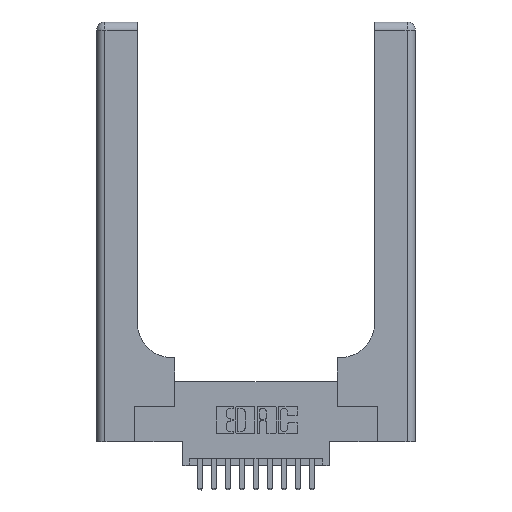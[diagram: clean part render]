
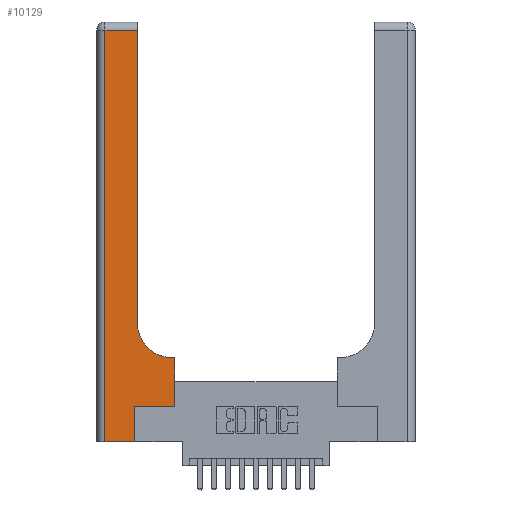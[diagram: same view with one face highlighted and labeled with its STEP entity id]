
A CAD part, top view. The second image highlights one B-rep face of the part: STEP entity #10129.
In plain terms, the highlighted planar face has unit normal (0, 0, 1).
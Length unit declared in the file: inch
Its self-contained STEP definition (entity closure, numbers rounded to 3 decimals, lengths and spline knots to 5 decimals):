
#326 = EDGE_CURVE ( 'NONE', #15477, #10815, #2946, .T. ) ;
#1832 = VECTOR ( 'NONE', #1956, 39.37008 ) ;
#1858 = LINE ( 'NONE', #14851, #14937 ) ;
#1953 = CARTESIAN_POINT ( 'NONE',  ( 0.2915, 0.85, 0.37 ) ) ;
#1956 = DIRECTION ( 'NONE',  ( 0., 1., 0. ) ) ;
#2002 = CARTESIAN_POINT ( 'NONE',  ( 0.2915, 0.6, 0.37 ) ) ;
#2609 = EDGE_CURVE ( 'NONE', #10669, #10481, #1858, .T. ) ;
#2946 = CIRCLE ( 'NONE', #4469, 0.25 ) ;
#3110 = CARTESIAN_POINT ( 'NONE',  ( 0.269, 0., 0.37 ) ) ;
#3187 = LINE ( 'NONE', #10203, #13603 ) ;
#3251 = DIRECTION ( 'NONE',  ( -1., 0., 0. ) ) ;
#3712 = CARTESIAN_POINT ( 'NONE',  ( 0.06, 3., 0.37 ) ) ;
#3766 = ORIENTED_EDGE ( 'NONE', *, *, #4899, .T. ) ;
#3911 = FACE_OUTER_BOUND ( 'NONE', #16599, .T. ) ;
#4209 = VECTOR ( 'NONE', #14157, 39.37008 ) ;
#4416 = LINE ( 'NONE', #11910, #14427 ) ;
#4467 = EDGE_CURVE ( 'NONE', #6904, #6610, #9529, .T. ) ;
#4469 = AXIS2_PLACEMENT_3D ( 'NONE', #9163, #15567, #6427 ) ;
#4899 = EDGE_CURVE ( 'NONE', #5593, #10669, #9102, .T. ) ;
#5244 = DIRECTION ( 'NONE',  ( 0., 1., 0. ) ) ;
#5484 = LINE ( 'NONE', #11302, #1832 ) ;
#5593 = VERTEX_POINT ( 'NONE', #8264 ) ;
#5919 = CARTESIAN_POINT ( 'NONE',  ( 0.5585, 0.6, 0.37 ) ) ;
#6427 = DIRECTION ( 'NONE',  ( 1., 0., 0. ) ) ;
#6610 = VERTEX_POINT ( 'NONE', #9978 ) ;
#6904 = VERTEX_POINT ( 'NONE', #7119 ) ;
#6950 = DIRECTION ( 'NONE',  ( 1., 0., 0. ) ) ;
#7119 = CARTESIAN_POINT ( 'NONE',  ( 0.269, 0.25, 0.37 ) ) ;
#7293 = EDGE_CURVE ( 'NONE', #10815, #11517, #3187, .T. ) ;
#7349 = DIRECTION ( 'NONE',  ( -1., 0., 0. ) ) ;
#7814 = EDGE_CURVE ( 'NONE', #15400, #15477, #13588, .T. ) ;
#7849 = ORIENTED_EDGE ( 'NONE', *, *, #12484, .T. ) ;
#8144 = CARTESIAN_POINT ( 'NONE',  ( 0.269, 0.25, 0.37 ) ) ;
#8264 = CARTESIAN_POINT ( 'NONE',  ( 0.06, 2.94, 0.37 ) ) ;
#8269 = ORIENTED_EDGE ( 'NONE', *, *, #15167, .T. ) ;
#8427 = DIRECTION ( 'NONE',  ( 0., 1., 0. ) ) ;
#8484 = CARTESIAN_POINT ( 'NONE',  ( 0.5415, 0.6, 0.37 ) ) ;
#8886 = LINE ( 'NONE', #11051, #14411 ) ;
#9054 = DIRECTION ( 'NONE',  ( -1., 0., 0. ) ) ;
#9102 = LINE ( 'NONE', #3712, #4209 ) ;
#9163 = CARTESIAN_POINT ( 'NONE',  ( 0.5415, 0.85, 0.37 ) ) ;
#9529 = LINE ( 'NONE', #8144, #13020 ) ;
#9637 = CARTESIAN_POINT ( 'NONE',  ( 0., 3., 0.37 ) ) ;
#9913 = AXIS2_PLACEMENT_3D ( 'NONE', #9637, #11069, #3251 ) ;
#9978 = CARTESIAN_POINT ( 'NONE',  ( 0.5585, 0.25, 0.37 ) ) ;
#10129 = ADVANCED_FACE ( 'NONE', ( #3911 ), #12231, .F. ) ;
#10203 = CARTESIAN_POINT ( 'NONE',  ( 0.2915, 3., 0.37 ) ) ;
#10481 = VERTEX_POINT ( 'NONE', #3110 ) ;
#10669 = VERTEX_POINT ( 'NONE', #12006 ) ;
#10707 = ORIENTED_EDGE ( 'NONE', *, *, #15401, .T. ) ;
#10815 = VERTEX_POINT ( 'NONE', #1953 ) ;
#11051 = CARTESIAN_POINT ( 'NONE',  ( 0.269, 0., 0.37 ) ) ;
#11069 = DIRECTION ( 'NONE',  ( 0., 0., -1. ) ) ;
#11302 = CARTESIAN_POINT ( 'NONE',  ( 0.5585, 0.25, 0.37 ) ) ;
#11452 = CARTESIAN_POINT ( 'NONE',  ( 0.2915, 2.94, 0.37 ) ) ;
#11488 = ORIENTED_EDGE ( 'NONE', *, *, #7293, .T. ) ;
#11517 = VERTEX_POINT ( 'NONE', #11452 ) ;
#11910 = CARTESIAN_POINT ( 'NONE',  ( 0., 2.94, 0.37 ) ) ;
#12006 = CARTESIAN_POINT ( 'NONE',  ( 0.06, 0., 0.37 ) ) ;
#12052 = ORIENTED_EDGE ( 'NONE', *, *, #2609, .T. ) ;
#12231 = PLANE ( 'NONE',  #9913 ) ;
#12484 = EDGE_CURVE ( 'NONE', #6610, #15400, #5484, .T. ) ;
#13020 = VECTOR ( 'NONE', #6950, 39.37008 ) ;
#13050 = ORIENTED_EDGE ( 'NONE', *, *, #7814, .T. ) ;
#13588 = LINE ( 'NONE', #2002, #16691 ) ;
#13603 = VECTOR ( 'NONE', #5244, 39.37008 ) ;
#13664 = ORIENTED_EDGE ( 'NONE', *, *, #326, .T. ) ;
#14157 = DIRECTION ( 'NONE',  ( 0., -1., 0. ) ) ;
#14411 = VECTOR ( 'NONE', #8427, 39.37008 ) ;
#14427 = VECTOR ( 'NONE', #9054, 39.37008 ) ;
#14737 = ORIENTED_EDGE ( 'NONE', *, *, #4467, .T. ) ;
#14793 = DIRECTION ( 'NONE',  ( 1., 0., 0. ) ) ;
#14851 = CARTESIAN_POINT ( 'NONE',  ( 0., 0., 0.37 ) ) ;
#14937 = VECTOR ( 'NONE', #14793, 39.37008 ) ;
#15167 = EDGE_CURVE ( 'NONE', #11517, #5593, #4416, .T. ) ;
#15400 = VERTEX_POINT ( 'NONE', #5919 ) ;
#15401 = EDGE_CURVE ( 'NONE', #10481, #6904, #8886, .T. ) ;
#15477 = VERTEX_POINT ( 'NONE', #8484 ) ;
#15567 = DIRECTION ( 'NONE',  ( 0., 0., -1. ) ) ;
#16599 = EDGE_LOOP ( 'NONE', ( #11488, #8269, #3766, #12052, #10707, #14737, #7849, #13050, #13664 ) ) ;
#16691 = VECTOR ( 'NONE', #7349, 39.37008 ) ;
